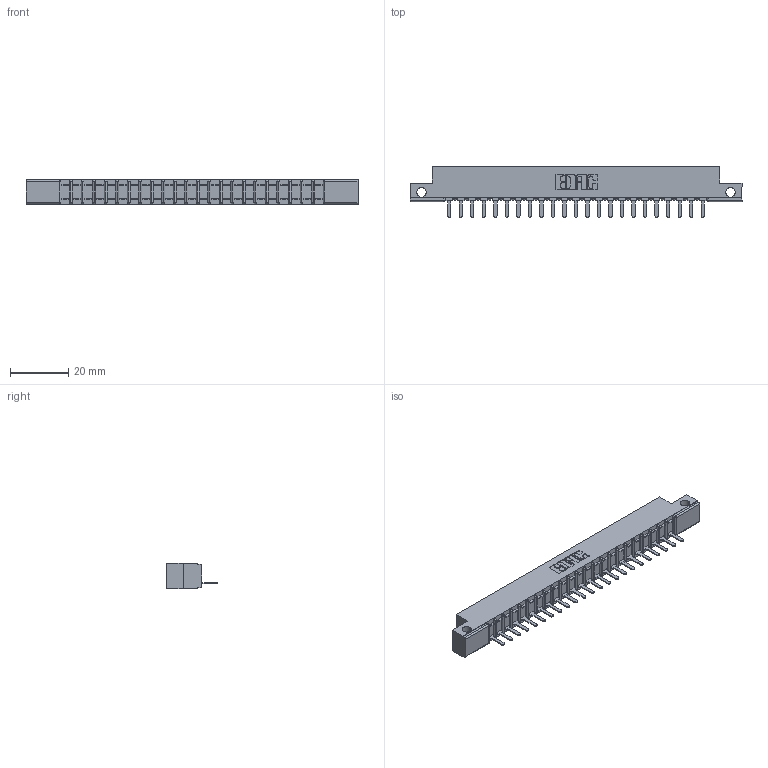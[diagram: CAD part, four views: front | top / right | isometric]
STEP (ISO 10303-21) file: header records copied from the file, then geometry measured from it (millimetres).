
FILE_DESCRIPTION (( 'STEP AP203' ), '1' );
FILE_NAME ('307-023-521-112.STEP', '2018-08-04T05:23:30', ( '' ), ( '' ), 'SwSTEP 2.0', 'SolidWorks 2016', '' );
FILE_SCHEMA (( 'CONFIG_CONTROL_DESIGN' ));
Length unit declared in the file: inch
Products named in the file (3): 307 Part_.128 Dia Side Mounting Holes; 307-290-002_521; 307-023-521-112
Assembly tree (24 placements, depth 2):
  307-023-521-112
    307 Part_.128 Dia Side Mounting Holes
    307-290-002_521  x23
Bounding box: 114.15 x 17.42 x 8.71 mm (x, y, z)
Volume: 7461.8 mm3; surface area: 13503.5 mm2
Topology: 24 solids, 24 shells, 1844 faces, 5659 edges, 3706 vertices
Faces by surface type: plane 1105, cylinder 691, sphere 48
Entity records: 22780 total; most frequent: CARTESIAN_POINT 3840, ORIENTED_EDGE 3830, DIRECTION 3739, EDGE_CURVE 1915, VECTOR 1457, LINE 1457, VERTEX_POINT 1242, AXIS2_PLACEMENT_3D 1141
